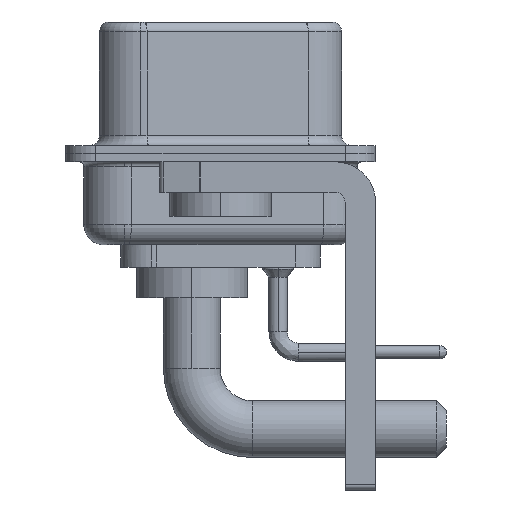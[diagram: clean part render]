
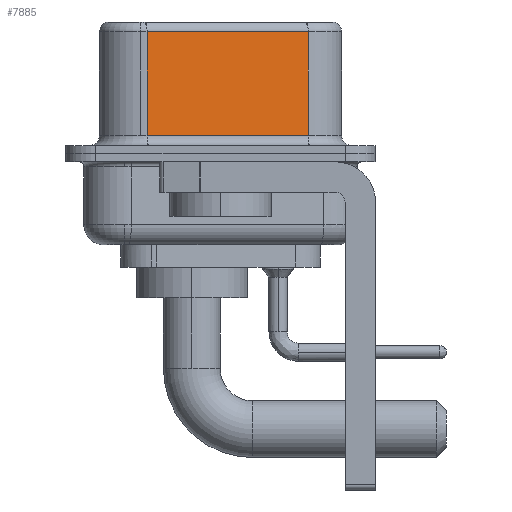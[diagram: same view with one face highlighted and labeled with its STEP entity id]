
A CAD part, left-side view. The second image highlights one B-rep face of the part: STEP entity #7885.
In plain terms, the highlighted planar face has unit normal (-0.985, -0.174, 0).
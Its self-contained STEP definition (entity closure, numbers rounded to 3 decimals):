
#606 = ORIENTED_EDGE ( 'NONE', *, *, #18870, .T. ) ;
#717 = DIRECTION ( 'NONE',  ( -0.174, 0.985, 0. ) ) ;
#1044 = VECTOR ( 'NONE', #6017, 1000. ) ;
#1093 = DIRECTION ( 'NONE',  ( 0.985, 0.174, 0. ) ) ;
#1129 = CARTESIAN_POINT ( 'NONE',  ( 5.132, -4.322, 6.02 ) ) ;
#2987 = FACE_OUTER_BOUND ( 'NONE', #7925, .T. ) ;
#4061 = LINE ( 'NONE', #11859, #10698 ) ;
#4456 = VERTEX_POINT ( 'NONE', #7364 ) ;
#5310 = ORIENTED_EDGE ( 'NONE', *, *, #8507, .T. ) ;
#6017 = DIRECTION ( 'NONE',  ( -0.174, 0.985, 0. ) ) ;
#6512 = VECTOR ( 'NONE', #22736, 1000. ) ;
#6991 = VECTOR ( 'NONE', #20289, 1000. ) ;
#7364 = CARTESIAN_POINT ( 'NONE',  ( 3.73, 3.628, 6.02 ) ) ;
#7750 = ORIENTED_EDGE ( 'NONE', *, *, #12946, .T. ) ;
#7885 = ADVANCED_FACE ( 'NONE', ( #2987 ), #14177, .F. ) ;
#7925 = EDGE_LOOP ( 'NONE', ( #19460, #606, #7750, #5310 ) ) ;
#8507 = EDGE_CURVE ( 'NONE', #17392, #19605, #4061, .T. ) ;
#9727 = LINE ( 'NONE', #15360, #6512 ) ;
#10698 = VECTOR ( 'NONE', #15844, 1000. ) ;
#11859 = CARTESIAN_POINT ( 'NONE',  ( 5.132, -4.322, 0.9 ) ) ;
#12683 = CARTESIAN_POINT ( 'NONE',  ( 5.132, -4.322, 6.52 ) ) ;
#12946 = EDGE_CURVE ( 'NONE', #4456, #17392, #9727, .T. ) ;
#14177 = PLANE ( 'NONE',  #21457 ) ;
#14227 = CARTESIAN_POINT ( 'NONE',  ( 5.132, -4.322, 0.9 ) ) ;
#14721 = EDGE_CURVE ( 'NONE', #20432, #19605, #22180, .T. ) ;
#15360 = CARTESIAN_POINT ( 'NONE',  ( 3.73, 3.628, 6.52 ) ) ;
#15844 = DIRECTION ( 'NONE',  ( 0.174, -0.985, 0. ) ) ;
#17392 = VERTEX_POINT ( 'NONE', #19879 ) ;
#18306 = CARTESIAN_POINT ( 'NONE',  ( 5.132, -4.322, 6.52 ) ) ;
#18870 = EDGE_CURVE ( 'NONE', #20432, #4456, #24334, .T. ) ;
#19460 = ORIENTED_EDGE ( 'NONE', *, *, #14721, .F. ) ;
#19605 = VERTEX_POINT ( 'NONE', #14227 ) ;
#19879 = CARTESIAN_POINT ( 'NONE',  ( 3.73, 3.628, 0.9 ) ) ;
#20289 = DIRECTION ( 'NONE',  ( 0., 0., -1. ) ) ;
#20432 = VERTEX_POINT ( 'NONE', #1129 ) ;
#21434 = CARTESIAN_POINT ( 'NONE',  ( 5.132, -4.322, 6.02 ) ) ;
#21457 = AXIS2_PLACEMENT_3D ( 'NONE', #18306, #1093, #717 ) ;
#22180 = LINE ( 'NONE', #12683, #6991 ) ;
#22736 = DIRECTION ( 'NONE',  ( 0., 0., -1. ) ) ;
#24334 = LINE ( 'NONE', #21434, #1044 ) ;
